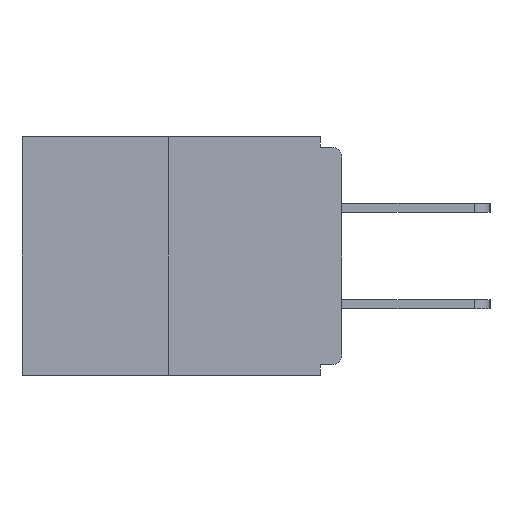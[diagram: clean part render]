
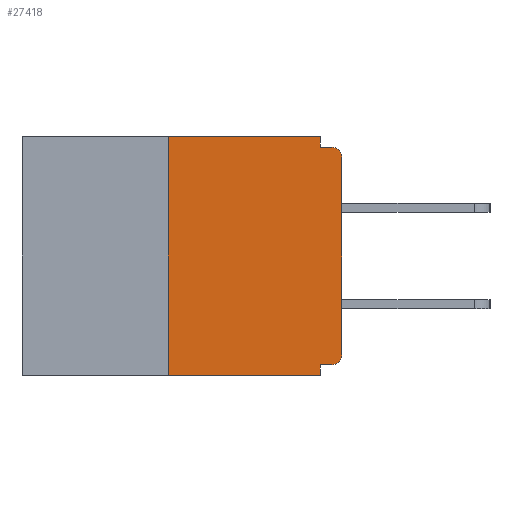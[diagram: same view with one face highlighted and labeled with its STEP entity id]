
A CAD part, left-side view. The second image highlights one B-rep face of the part: STEP entity #27418.
In plain terms, the highlighted planar face has unit normal (-1, 0, 0).
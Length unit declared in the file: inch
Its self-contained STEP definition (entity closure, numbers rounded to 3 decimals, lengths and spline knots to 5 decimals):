
#148 = AXIS2_PLACEMENT_3D ( 'NONE', #6792, #15520, #11233 ) ;
#754 = CIRCLE ( 'NONE', #148, 0.015 ) ;
#1073 = CARTESIAN_POINT ( 'NONE',  ( 0., 0.031, 0. ) ) ;
#1396 = EDGE_CURVE ( 'NONE', #21645, #19965, #754, .T. ) ;
#1520 = ORIENTED_EDGE ( 'NONE', *, *, #21709, .T. ) ;
#1767 = DIRECTION ( 'NONE',  ( -1., 0., 0. ) ) ;
#1851 = VERTEX_POINT ( 'NONE', #6478 ) ;
#2652 = CARTESIAN_POINT ( 'NONE',  ( 0., 0.015, -0.015 ) ) ;
#2700 = DIRECTION ( 'NONE',  ( 0., 0., -1. ) ) ;
#2706 = DIRECTION ( 'NONE',  ( 0., -1., 0. ) ) ;
#2858 = EDGE_CURVE ( 'NONE', #18636, #14544, #9686, .T. ) ;
#2932 = DIRECTION ( 'NONE',  ( 0., 0., -1. ) ) ;
#3174 = LINE ( 'NONE', #23563, #23755 ) ;
#3650 = EDGE_CURVE ( 'NONE', #26165, #15328, #9283, .T. ) ;
#3786 = CIRCLE ( 'NONE', #21418, 0.015 ) ;
#3951 = ORIENTED_EDGE ( 'NONE', *, *, #22328, .F. ) ;
#4466 = VECTOR ( 'NONE', #2706, 39.37008 ) ;
#5219 = EDGE_CURVE ( 'NONE', #15274, #26165, #6094, .T. ) ;
#5333 = DIRECTION ( 'NONE',  ( 0., 1., 0. ) ) ;
#5441 = CARTESIAN_POINT ( 'NONE',  ( 0., 0.25, -0.343 ) ) ;
#6094 = LINE ( 'NONE', #23694, #13319 ) ;
#6478 = CARTESIAN_POINT ( 'NONE',  ( 0., 0.031, -0.328 ) ) ;
#6493 = DIRECTION ( 'NONE',  ( 0., 0., -1. ) ) ;
#6792 = CARTESIAN_POINT ( 'NONE',  ( 0., 0.015, -0.313 ) ) ;
#7504 = CARTESIAN_POINT ( 'NONE',  ( 0., 0.031, -0.015 ) ) ;
#8741 = CARTESIAN_POINT ( 'NONE',  ( 0., 0.031, -0.343 ) ) ;
#8983 = CARTESIAN_POINT ( 'NONE',  ( 0., 0.031, 0. ) ) ;
#9117 = CARTESIAN_POINT ( 'NONE',  ( 0., 0., -0.03 ) ) ;
#9283 = LINE ( 'NONE', #15646, #4466 ) ;
#9479 = CARTESIAN_POINT ( 'NONE',  ( 0., 0.015, -0.328 ) ) ;
#9489 = PLANE ( 'NONE',  #18073 ) ;
#9686 = LINE ( 'NONE', #13930, #25142 ) ;
#9746 = ORIENTED_EDGE ( 'NONE', *, *, #17629, .F. ) ;
#10482 = EDGE_CURVE ( 'NONE', #21645, #1851, #20610, .T. ) ;
#11233 = DIRECTION ( 'NONE',  ( 0., 0., -1. ) ) ;
#11825 = DIRECTION ( 'NONE',  ( 1., 0., 0. ) ) ;
#12511 = FACE_OUTER_BOUND ( 'NONE', #14053, .T. ) ;
#13319 = VECTOR ( 'NONE', #28102, 39.37008 ) ;
#13677 = CARTESIAN_POINT ( 'NONE',  ( 0., 0., -0.313 ) ) ;
#13903 = DIRECTION ( 'NONE',  ( 0., 0., -1. ) ) ;
#13930 = CARTESIAN_POINT ( 'NONE',  ( 0., 0., -0.015 ) ) ;
#14053 = EDGE_LOOP ( 'NONE', ( #21917, #21611, #19569, #9746, #15042, #26950, #1520, #16104, #25747, #3951 ) ) ;
#14458 = VECTOR ( 'NONE', #6493, 39.37008 ) ;
#14544 = VERTEX_POINT ( 'NONE', #2652 ) ;
#15042 = ORIENTED_EDGE ( 'NONE', *, *, #10482, .F. ) ;
#15274 = VERTEX_POINT ( 'NONE', #5441 ) ;
#15328 = VERTEX_POINT ( 'NONE', #1073 ) ;
#15408 = VECTOR ( 'NONE', #2700, 39.37008 ) ;
#15520 = DIRECTION ( 'NONE',  ( -1., 0., 0. ) ) ;
#15646 = CARTESIAN_POINT ( 'NONE',  ( 0., 0.46, 0. ) ) ;
#15784 = DIRECTION ( 'NONE',  ( 0., -1., 0. ) ) ;
#16104 = ORIENTED_EDGE ( 'NONE', *, *, #16884, .T. ) ;
#16506 = CARTESIAN_POINT ( 'NONE',  ( 0., 0.25, 0. ) ) ;
#16884 = EDGE_CURVE ( 'NONE', #17657, #14544, #3786, .T. ) ;
#17629 = EDGE_CURVE ( 'NONE', #1851, #22686, #20557, .T. ) ;
#17657 = VERTEX_POINT ( 'NONE', #9117 ) ;
#17746 = LINE ( 'NONE', #26516, #27734 ) ;
#18073 = AXIS2_PLACEMENT_3D ( 'NONE', #25022, #11825, #13903 ) ;
#18636 = VERTEX_POINT ( 'NONE', #7504 ) ;
#19115 = CARTESIAN_POINT ( 'NONE',  ( 0., 0.031, -0.343 ) ) ;
#19209 = DIRECTION ( 'NONE',  ( 0., 0., 1. ) ) ;
#19569 = ORIENTED_EDGE ( 'NONE', *, *, #28480, .T. ) ;
#19965 = VERTEX_POINT ( 'NONE', #13677 ) ;
#20557 = LINE ( 'NONE', #8741, #15408 ) ;
#20610 = LINE ( 'NONE', #22677, #28166 ) ;
#21418 = AXIS2_PLACEMENT_3D ( 'NONE', #25844, #1767, #2932 ) ;
#21611 = ORIENTED_EDGE ( 'NONE', *, *, #5219, .F. ) ;
#21645 = VERTEX_POINT ( 'NONE', #9479 ) ;
#21709 = EDGE_CURVE ( 'NONE', #19965, #17657, #3174, .T. ) ;
#21917 = ORIENTED_EDGE ( 'NONE', *, *, #3650, .F. ) ;
#22328 = EDGE_CURVE ( 'NONE', #15328, #18636, #23367, .T. ) ;
#22677 = CARTESIAN_POINT ( 'NONE',  ( 0., 0., -0.328 ) ) ;
#22686 = VERTEX_POINT ( 'NONE', #19115 ) ;
#23367 = LINE ( 'NONE', #8983, #14458 ) ;
#23563 = CARTESIAN_POINT ( 'NONE',  ( 0., 0., 0. ) ) ;
#23694 = CARTESIAN_POINT ( 'NONE',  ( 0., 0.25, 0. ) ) ;
#23755 = VECTOR ( 'NONE', #19209, 39.37008 ) ;
#25022 = CARTESIAN_POINT ( 'NONE',  ( 0., 0.46, 0. ) ) ;
#25142 = VECTOR ( 'NONE', #25143, 39.37008 ) ;
#25143 = DIRECTION ( 'NONE',  ( 0., -1., 0. ) ) ;
#25747 = ORIENTED_EDGE ( 'NONE', *, *, #2858, .F. ) ;
#25844 = CARTESIAN_POINT ( 'NONE',  ( 0., 0.015, -0.03 ) ) ;
#26165 = VERTEX_POINT ( 'NONE', #16506 ) ;
#26516 = CARTESIAN_POINT ( 'NONE',  ( 0., 0.46, -0.343 ) ) ;
#26950 = ORIENTED_EDGE ( 'NONE', *, *, #1396, .T. ) ;
#27418 = ADVANCED_FACE ( 'NONE', ( #12511 ), #9489, .F. ) ;
#27734 = VECTOR ( 'NONE', #15784, 39.37008 ) ;
#28102 = DIRECTION ( 'NONE',  ( 0., 0., 1. ) ) ;
#28166 = VECTOR ( 'NONE', #5333, 39.37008 ) ;
#28480 = EDGE_CURVE ( 'NONE', #15274, #22686, #17746, .T. ) ;
